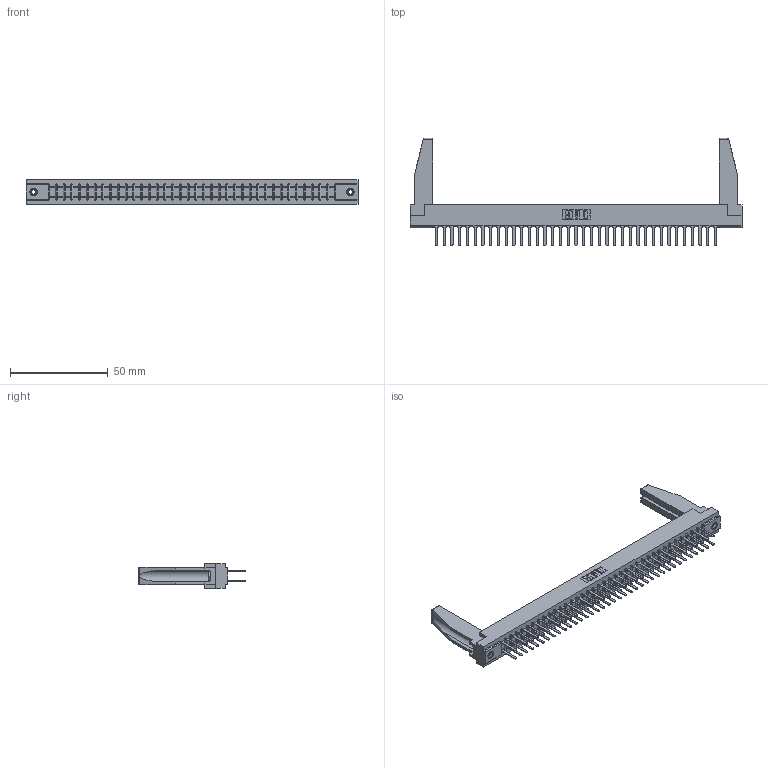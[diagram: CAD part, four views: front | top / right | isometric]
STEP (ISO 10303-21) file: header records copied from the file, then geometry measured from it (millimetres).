
FILE_DESCRIPTION (( 'STEP AP203' ), '1' );
FILE_NAME ('357-074-422-278.STEP', '2020-10-04T18:01:44', ( '' ), ( '' ), 'SwSTEP 2.0', 'SolidWorks 2020', '' );
FILE_SCHEMA (( 'CONFIG_CONTROL_DESIGN' ));
Length unit declared in the file: inch
Products named in the file (5): 357-074-422-278; 307-290-001_522; 307-220-078; 307 Part_.156 Dia Mounting Holes; 345-250-001_345-250-001-102
Assembly tree (79 placements, depth 2):
  357-074-422-278
    307 Part_.156 Dia Mounting Holes
    307-290-001_522  x74
    307-220-078  x2
    345-250-001_345-250-001-102  x2
Bounding box: 169.62 x 54.81 x 12.7 mm (x, y, z)
Volume: 22154.5 mm3; surface area: 26753.9 mm2
Topology: 79 solids, 79 shells, 3690 faces, 10273 edges, 6638 vertices
Faces by surface type: plane 2448, cylinder 1150, sphere 76, cone 12, torus 4
Entity records: 35927 total; most frequent: CARTESIAN_POINT 5887, ORIENTED_EDGE 5792, DIRECTION 5722, EDGE_CURVE 2896, LINE 2224, VECTOR 2224, VERTEX_POINT 1872, AXIS2_PLACEMENT_3D 1749
